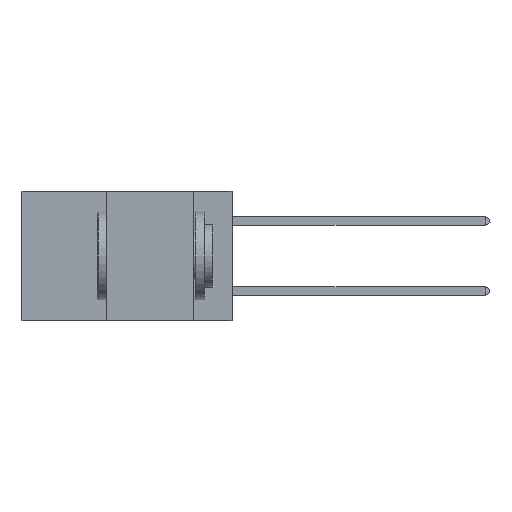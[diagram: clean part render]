
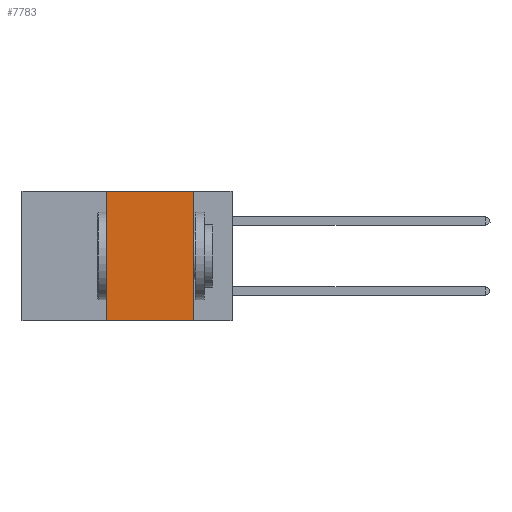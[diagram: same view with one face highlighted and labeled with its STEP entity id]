
A CAD part, left-side view. The second image highlights one B-rep face of the part: STEP entity #7783.
In plain terms, the highlighted planar face has unit normal (-1, 0, 0).
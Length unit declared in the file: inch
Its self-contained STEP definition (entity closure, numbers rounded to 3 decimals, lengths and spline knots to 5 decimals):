
#410 = DIRECTION ( 'NONE',  ( 1., 0., 0. ) ) ;
#412 = VERTEX_POINT ( 'NONE', #6861 ) ;
#486 = CARTESIAN_POINT ( 'NONE',  ( 0., 0.11, 0. ) ) ;
#769 = DIRECTION ( 'NONE',  ( 0., -1., 0. ) ) ;
#907 = LINE ( 'NONE', #5786, #10031 ) ;
#1079 = PLANE ( 'NONE',  #11146 ) ;
#2369 = CARTESIAN_POINT ( 'NONE',  ( 0., 0.11, -0.37 ) ) ;
#2392 = ORIENTED_EDGE ( 'NONE', *, *, #6212, .F. ) ;
#2871 = CARTESIAN_POINT ( 'NONE',  ( 0., 0.6, 0. ) ) ;
#2913 = EDGE_CURVE ( 'NONE', #9414, #5180, #9641, .T. ) ;
#3873 = DIRECTION ( 'NONE',  ( 0., 0., 1. ) ) ;
#4242 = VECTOR ( 'NONE', #769, 39.37008 ) ;
#4532 = LINE ( 'NONE', #7600, #9086 ) ;
#4646 = DIRECTION ( 'NONE',  ( 0., 0., -1. ) ) ;
#5065 = DIRECTION ( 'NONE',  ( 0., -1., 0. ) ) ;
#5105 = CARTESIAN_POINT ( 'NONE',  ( 0., 0.11, 0. ) ) ;
#5180 = VERTEX_POINT ( 'NONE', #486 ) ;
#5232 = FACE_OUTER_BOUND ( 'NONE', #7488, .T. ) ;
#5550 = CARTESIAN_POINT ( 'NONE',  ( 0., 0.36, 0. ) ) ;
#5786 = CARTESIAN_POINT ( 'NONE',  ( 0., 0.6, -0.37 ) ) ;
#6012 = CARTESIAN_POINT ( 'NONE',  ( 0., 0.6, 0. ) ) ;
#6212 = EDGE_CURVE ( 'NONE', #5180, #9744, #7295, .T. ) ;
#6504 = ORIENTED_EDGE ( 'NONE', *, *, #2913, .F. ) ;
#6761 = VECTOR ( 'NONE', #4646, 39.37008 ) ;
#6861 = CARTESIAN_POINT ( 'NONE',  ( 0., 0.36, -0.37 ) ) ;
#7295 = LINE ( 'NONE', #5105, #6761 ) ;
#7488 = EDGE_LOOP ( 'NONE', ( #2392, #6504, #10820, #8335 ) ) ;
#7600 = CARTESIAN_POINT ( 'NONE',  ( 0., 0.36, 0. ) ) ;
#7783 = ADVANCED_FACE ( 'NONE', ( #5232 ), #1079, .F. ) ;
#8267 = DIRECTION ( 'NONE',  ( 0., 0., -1. ) ) ;
#8335 = ORIENTED_EDGE ( 'NONE', *, *, #11010, .T. ) ;
#8629 = EDGE_CURVE ( 'NONE', #412, #9414, #4532, .T. ) ;
#9086 = VECTOR ( 'NONE', #3873, 39.37008 ) ;
#9414 = VERTEX_POINT ( 'NONE', #5550 ) ;
#9641 = LINE ( 'NONE', #6012, #4242 ) ;
#9744 = VERTEX_POINT ( 'NONE', #2369 ) ;
#10031 = VECTOR ( 'NONE', #5065, 39.37008 ) ;
#10820 = ORIENTED_EDGE ( 'NONE', *, *, #8629, .F. ) ;
#11010 = EDGE_CURVE ( 'NONE', #412, #9744, #907, .T. ) ;
#11146 = AXIS2_PLACEMENT_3D ( 'NONE', #2871, #410, #8267 ) ;
